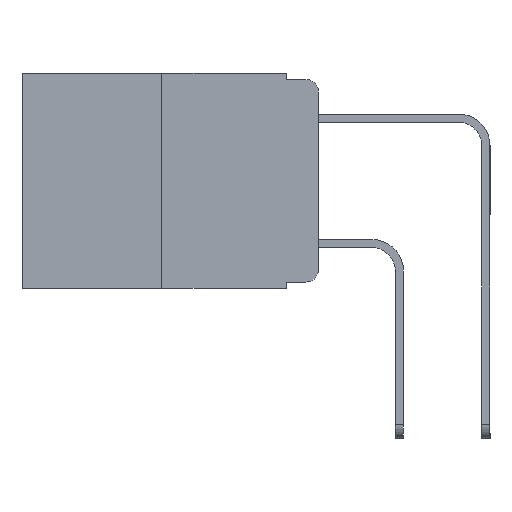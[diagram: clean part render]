
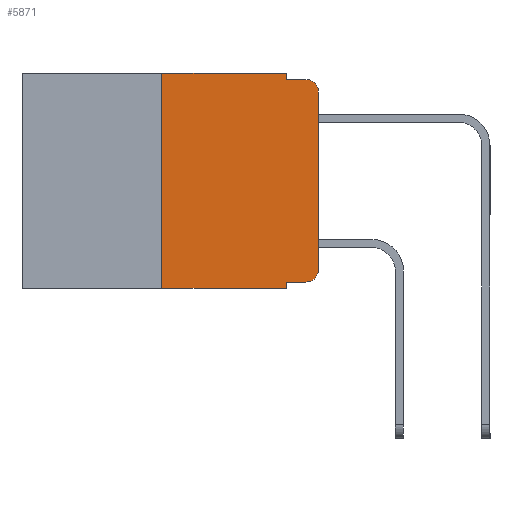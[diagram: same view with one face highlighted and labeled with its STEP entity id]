
A CAD part, left-side view. The second image highlights one B-rep face of the part: STEP entity #5871.
In plain terms, the highlighted planar face has unit normal (-1, 0, 0).
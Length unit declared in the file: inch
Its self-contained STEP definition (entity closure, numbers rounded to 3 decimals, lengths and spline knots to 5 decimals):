
#147 = CARTESIAN_POINT ( 'NONE',  ( 0., 0.051, -0.333 ) ) ;
#1241 = DIRECTION ( 'NONE',  ( 0., 0., -1. ) ) ;
#1344 = CARTESIAN_POINT ( 'NONE',  ( 0., 0.02, -0.333 ) ) ;
#1390 = VERTEX_POINT ( 'NONE', #22304 ) ;
#1588 = CARTESIAN_POINT ( 'NONE',  ( 0., 0.051, -0.01 ) ) ;
#2058 = CARTESIAN_POINT ( 'NONE',  ( 0., 0.25, 0. ) ) ;
#2225 = VERTEX_POINT ( 'NONE', #17052 ) ;
#2241 = ORIENTED_EDGE ( 'NONE', *, *, #13310, .T. ) ;
#3290 = ORIENTED_EDGE ( 'NONE', *, *, #24933, .T. ) ;
#3998 = DIRECTION ( 'NONE',  ( 0., 0., -1. ) ) ;
#4214 = CIRCLE ( 'NONE', #24809, 0.02 ) ;
#4291 = CARTESIAN_POINT ( 'NONE',  ( 0., 0.051, -0.01 ) ) ;
#4797 = VECTOR ( 'NONE', #25769, 39.37008 ) ;
#5174 = EDGE_CURVE ( 'NONE', #24127, #21843, #5313, .T. ) ;
#5313 = LINE ( 'NONE', #4291, #21509 ) ;
#5636 = ORIENTED_EDGE ( 'NONE', *, *, #9972, .F. ) ;
#5855 = VECTOR ( 'NONE', #25913, 39.37008 ) ;
#5871 = ADVANCED_FACE ( 'NONE', ( #16225 ), #8167, .F. ) ;
#6027 = DIRECTION ( 'NONE',  ( 0., -1., 0. ) ) ;
#6061 = CARTESIAN_POINT ( 'NONE',  ( 0., 0.051, -0.333 ) ) ;
#6254 = LINE ( 'NONE', #147, #11247 ) ;
#6377 = VERTEX_POINT ( 'NONE', #1344 ) ;
#6459 = VECTOR ( 'NONE', #24328, 39.37008 ) ;
#6475 = VECTOR ( 'NONE', #6027, 39.37008 ) ;
#6574 = DIRECTION ( 'NONE',  ( 0., 0., -1. ) ) ;
#6676 = DIRECTION ( 'NONE',  ( 0., -1., 0. ) ) ;
#7148 = VERTEX_POINT ( 'NONE', #6061 ) ;
#7459 = AXIS2_PLACEMENT_3D ( 'NONE', #26498, #13959, #1241 ) ;
#8167 = PLANE ( 'NONE',  #26723 ) ;
#8662 = CARTESIAN_POINT ( 'NONE',  ( 0., 0.02, -0.03 ) ) ;
#9041 = LINE ( 'NONE', #21336, #14658 ) ;
#9615 = CARTESIAN_POINT ( 'NONE',  ( 0., 0.051, 0. ) ) ;
#9728 = CARTESIAN_POINT ( 'NONE',  ( 0., 0.051, 0. ) ) ;
#9781 = VERTEX_POINT ( 'NONE', #16257 ) ;
#9972 = EDGE_CURVE ( 'NONE', #9781, #26951, #16271, .T. ) ;
#10389 = ORIENTED_EDGE ( 'NONE', *, *, #12463, .F. ) ;
#10453 = LINE ( 'NONE', #15362, #4797 ) ;
#10809 = DIRECTION ( 'NONE',  ( 0., 0., -1. ) ) ;
#11247 = VECTOR ( 'NONE', #6676, 39.37008 ) ;
#11473 = LINE ( 'NONE', #20810, #6475 ) ;
#12314 = EDGE_CURVE ( 'NONE', #2225, #21843, #4214, .T. ) ;
#12326 = ORIENTED_EDGE ( 'NONE', *, *, #12314, .T. ) ;
#12463 = EDGE_CURVE ( 'NONE', #26951, #19158, #23976, .T. ) ;
#12863 = ORIENTED_EDGE ( 'NONE', *, *, #15651, .F. ) ;
#13223 = ORIENTED_EDGE ( 'NONE', *, *, #23125, .T. ) ;
#13310 = EDGE_CURVE ( 'NONE', #9781, #1390, #11473, .T. ) ;
#13404 = VERTEX_POINT ( 'NONE', #25092 ) ;
#13959 = DIRECTION ( 'NONE',  ( -1., 0., 0. ) ) ;
#14547 = CARTESIAN_POINT ( 'NONE',  ( 0., 0.473, 0. ) ) ;
#14658 = VECTOR ( 'NONE', #6574, 39.37008 ) ;
#14866 = ORIENTED_EDGE ( 'NONE', *, *, #25090, .F. ) ;
#15125 = ORIENTED_EDGE ( 'NONE', *, *, #5174, .F. ) ;
#15362 = CARTESIAN_POINT ( 'NONE',  ( 0., 0., 0. ) ) ;
#15608 = VECTOR ( 'NONE', #27285, 39.37008 ) ;
#15628 = CARTESIAN_POINT ( 'NONE',  ( 0., 0.25, 0. ) ) ;
#15651 = EDGE_CURVE ( 'NONE', #19158, #24127, #9041, .T. ) ;
#16225 = FACE_OUTER_BOUND ( 'NONE', #25205, .T. ) ;
#16257 = CARTESIAN_POINT ( 'NONE',  ( 0., 0.25, -0.343 ) ) ;
#16271 = LINE ( 'NONE', #2058, #15608 ) ;
#16686 = DIRECTION ( 'NONE',  ( 1., 0., 0. ) ) ;
#17046 = LINE ( 'NONE', #9615, #6459 ) ;
#17052 = CARTESIAN_POINT ( 'NONE',  ( 0., 0., -0.03 ) ) ;
#17533 = CARTESIAN_POINT ( 'NONE',  ( 0., 0.473, 0. ) ) ;
#19158 = VERTEX_POINT ( 'NONE', #9728 ) ;
#20090 = CIRCLE ( 'NONE', #7459, 0.02 ) ;
#20810 = CARTESIAN_POINT ( 'NONE',  ( 0., 0.473, -0.343 ) ) ;
#21195 = DIRECTION ( 'NONE',  ( 0., -1., 0. ) ) ;
#21336 = CARTESIAN_POINT ( 'NONE',  ( 0., 0.051, 0. ) ) ;
#21509 = VECTOR ( 'NONE', #21195, 39.37008 ) ;
#21843 = VERTEX_POINT ( 'NONE', #25307 ) ;
#22304 = CARTESIAN_POINT ( 'NONE',  ( 0., 0.051, -0.343 ) ) ;
#23125 = EDGE_CURVE ( 'NONE', #7148, #6377, #6254, .T. ) ;
#23369 = DIRECTION ( 'NONE',  ( -1., 0., 0. ) ) ;
#23976 = LINE ( 'NONE', #17533, #5855 ) ;
#24127 = VERTEX_POINT ( 'NONE', #1588 ) ;
#24328 = DIRECTION ( 'NONE',  ( 0., 0., -1. ) ) ;
#24809 = AXIS2_PLACEMENT_3D ( 'NONE', #8662, #23369, #10809 ) ;
#24933 = EDGE_CURVE ( 'NONE', #13404, #2225, #10453, .T. ) ;
#25090 = EDGE_CURVE ( 'NONE', #7148, #1390, #17046, .T. ) ;
#25092 = CARTESIAN_POINT ( 'NONE',  ( 0., 0., -0.313 ) ) ;
#25205 = EDGE_LOOP ( 'NONE', ( #3290, #12326, #15125, #12863, #10389, #5636, #2241, #14866, #13223, #26693 ) ) ;
#25307 = CARTESIAN_POINT ( 'NONE',  ( 0., 0.02, -0.01 ) ) ;
#25769 = DIRECTION ( 'NONE',  ( 0., 0., 1. ) ) ;
#25913 = DIRECTION ( 'NONE',  ( 0., -1., 0. ) ) ;
#26498 = CARTESIAN_POINT ( 'NONE',  ( 0., 0.02, -0.313 ) ) ;
#26693 = ORIENTED_EDGE ( 'NONE', *, *, #27074, .T. ) ;
#26723 = AXIS2_PLACEMENT_3D ( 'NONE', #14547, #16686, #3998 ) ;
#26951 = VERTEX_POINT ( 'NONE', #15628 ) ;
#27074 = EDGE_CURVE ( 'NONE', #6377, #13404, #20090, .T. ) ;
#27285 = DIRECTION ( 'NONE',  ( 0., 0., 1. ) ) ;
